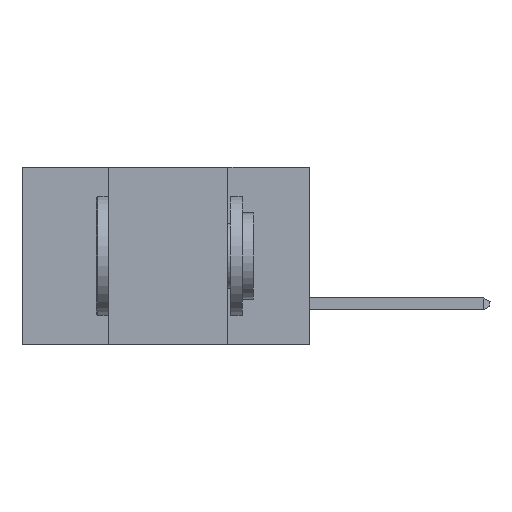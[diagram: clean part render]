
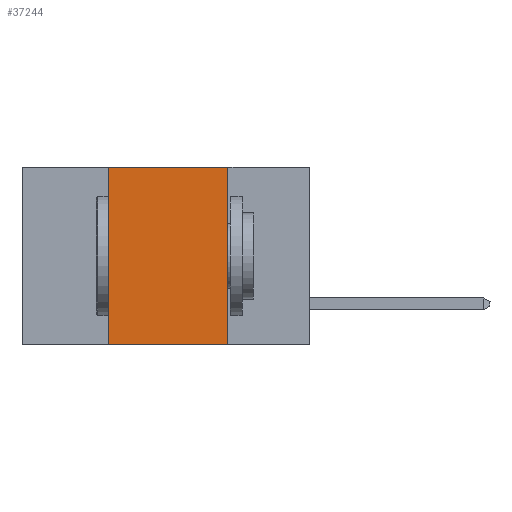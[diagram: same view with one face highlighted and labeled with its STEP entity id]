
A CAD part, left-side view. The second image highlights one B-rep face of the part: STEP entity #37244.
In plain terms, the highlighted planar face has unit normal (-1, 0, 0).
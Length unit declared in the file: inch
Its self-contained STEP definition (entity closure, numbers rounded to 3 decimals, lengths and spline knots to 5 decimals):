
#1712 = ORIENTED_EDGE ( 'NONE', *, *, #32022, .F. ) ;
#3210 = DIRECTION ( 'NONE',  ( 0., 0., -1. ) ) ;
#7324 = EDGE_CURVE ( 'NONE', #20382, #16483, #38328, .T. ) ;
#7734 = CARTESIAN_POINT ( 'NONE',  ( 0., 0.42, 0. ) ) ;
#10343 = EDGE_CURVE ( 'NONE', #25333, #28562, #45938, .T. ) ;
#13873 = CARTESIAN_POINT ( 'NONE',  ( 0., 0.17, 0. ) ) ;
#15116 = ORIENTED_EDGE ( 'NONE', *, *, #10343, .F. ) ;
#16013 = CARTESIAN_POINT ( 'NONE',  ( 0., 0.17, -0.37 ) ) ;
#16483 = VERTEX_POINT ( 'NONE', #16013 ) ;
#17120 = DIRECTION ( 'NONE',  ( 0., -1., 0. ) ) ;
#17756 = DIRECTION ( 'NONE',  ( 1., 0., 0. ) ) ;
#18076 = EDGE_CURVE ( 'NONE', #20382, #25333, #30983, .T. ) ;
#18689 = AXIS2_PLACEMENT_3D ( 'NONE', #43534, #17756, #3210 ) ;
#20382 = VERTEX_POINT ( 'NONE', #35715 ) ;
#21064 = ORIENTED_EDGE ( 'NONE', *, *, #18076, .F. ) ;
#21296 = VECTOR ( 'NONE', #28368, 39.37008 ) ;
#21395 = VECTOR ( 'NONE', #40336, 39.37008 ) ;
#23883 = VECTOR ( 'NONE', #25323, 39.37008 ) ;
#25323 = DIRECTION ( 'NONE',  ( 0., 0., -1. ) ) ;
#25333 = VERTEX_POINT ( 'NONE', #7734 ) ;
#26033 = CARTESIAN_POINT ( 'NONE',  ( 0., 0.6, 0. ) ) ;
#28368 = DIRECTION ( 'NONE',  ( 0., 0., 1. ) ) ;
#28531 = CARTESIAN_POINT ( 'NONE',  ( 0., 0.42, 0. ) ) ;
#28562 = VERTEX_POINT ( 'NONE', #45962 ) ;
#30983 = LINE ( 'NONE', #28531, #21296 ) ;
#32022 = EDGE_CURVE ( 'NONE', #28562, #16483, #46721, .T. ) ;
#35715 = CARTESIAN_POINT ( 'NONE',  ( 0., 0.42, -0.37 ) ) ;
#37244 = ADVANCED_FACE ( 'NONE', ( #41981 ), #39535, .F. ) ;
#38229 = EDGE_LOOP ( 'NONE', ( #1712, #15116, #21064, #44696 ) ) ;
#38328 = LINE ( 'NONE', #46261, #41753 ) ;
#39535 = PLANE ( 'NONE',  #18689 ) ;
#40336 = DIRECTION ( 'NONE',  ( 0., -1., 0. ) ) ;
#41753 = VECTOR ( 'NONE', #17120, 39.37008 ) ;
#41981 = FACE_OUTER_BOUND ( 'NONE', #38229, .T. ) ;
#43534 = CARTESIAN_POINT ( 'NONE',  ( 0., 0.6, 0. ) ) ;
#44696 = ORIENTED_EDGE ( 'NONE', *, *, #7324, .T. ) ;
#45938 = LINE ( 'NONE', #26033, #21395 ) ;
#45962 = CARTESIAN_POINT ( 'NONE',  ( 0., 0.17, 0. ) ) ;
#46261 = CARTESIAN_POINT ( 'NONE',  ( 0., 0.6, -0.37 ) ) ;
#46721 = LINE ( 'NONE', #13873, #23883 ) ;
